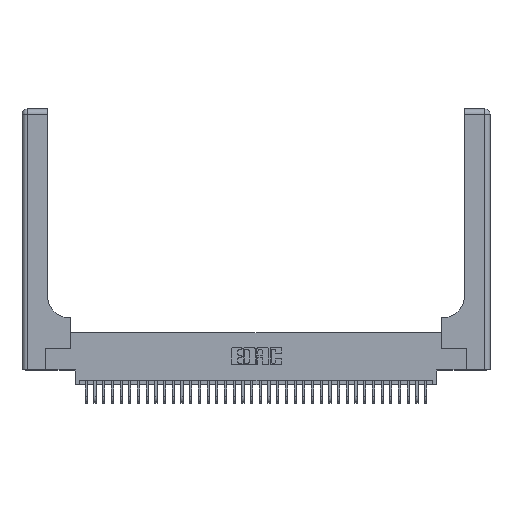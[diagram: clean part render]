
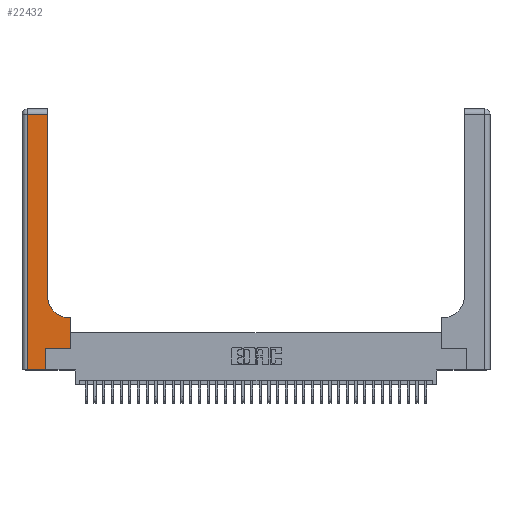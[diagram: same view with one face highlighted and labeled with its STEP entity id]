
A CAD part, top view. The second image highlights one B-rep face of the part: STEP entity #22432.
In plain terms, the highlighted planar face has unit normal (0, 0, 1).
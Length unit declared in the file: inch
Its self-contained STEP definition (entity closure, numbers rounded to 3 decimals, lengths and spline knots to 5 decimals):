
#737 = LINE ( 'NONE', #9791, #32551 ) ;
#1546 = VERTEX_POINT ( 'NONE', #38609 ) ;
#1738 = CARTESIAN_POINT ( 'NONE',  ( 0.5585, 0.25, 0.37 ) ) ;
#2170 = VERTEX_POINT ( 'NONE', #7391 ) ;
#2420 = ORIENTED_EDGE ( 'NONE', *, *, #10129, .T. ) ;
#2819 = CARTESIAN_POINT ( 'NONE',  ( 0., 3., 0.37 ) ) ;
#3541 = ORIENTED_EDGE ( 'NONE', *, *, #13930, .T. ) ;
#3680 = DIRECTION ( 'NONE',  ( -1., 0., 0. ) ) ;
#3943 = VECTOR ( 'NONE', #24016, 39.37008 ) ;
#4893 = LINE ( 'NONE', #12239, #3943 ) ;
#5303 = VECTOR ( 'NONE', #13798, 39.37008 ) ;
#5900 = DIRECTION ( 'NONE',  ( -1., 0., 0. ) ) ;
#5926 = EDGE_LOOP ( 'NONE', ( #15578, #2420, #13577, #8033, #20537, #35206, #3541, #31419, #14170 ) ) ;
#6678 = VECTOR ( 'NONE', #29207, 39.37008 ) ;
#7329 = AXIS2_PLACEMENT_3D ( 'NONE', #15722, #36368, #18679 ) ;
#7391 = CARTESIAN_POINT ( 'NONE',  ( 0.06, 0., 0.37 ) ) ;
#7452 = VERTEX_POINT ( 'NONE', #28634 ) ;
#7682 = CARTESIAN_POINT ( 'NONE',  ( 0.2915, 3., 0.37 ) ) ;
#8033 = ORIENTED_EDGE ( 'NONE', *, *, #23792, .T. ) ;
#9218 = CARTESIAN_POINT ( 'NONE',  ( 0.269, 0.25, 0.37 ) ) ;
#9411 = LINE ( 'NONE', #7682, #25226 ) ;
#9791 = CARTESIAN_POINT ( 'NONE',  ( 0., 2.94, 0.37 ) ) ;
#10129 = EDGE_CURVE ( 'NONE', #33311, #28318, #737, .T. ) ;
#11507 = CIRCLE ( 'NONE', #7329, 0.25 ) ;
#12239 = CARTESIAN_POINT ( 'NONE',  ( 0.269, 0., 0.37 ) ) ;
#13577 = ORIENTED_EDGE ( 'NONE', *, *, #18171, .T. ) ;
#13798 = DIRECTION ( 'NONE',  ( 0., 1., 0. ) ) ;
#13930 = EDGE_CURVE ( 'NONE', #38083, #7452, #28159, .T. ) ;
#14170 = ORIENTED_EDGE ( 'NONE', *, *, #38014, .T. ) ;
#14702 = LINE ( 'NONE', #26218, #6678 ) ;
#15578 = ORIENTED_EDGE ( 'NONE', *, *, #23328, .T. ) ;
#15722 = CARTESIAN_POINT ( 'NONE',  ( 0.5415, 0.85, 0.37 ) ) ;
#16207 = CARTESIAN_POINT ( 'NONE',  ( 0.06, 3., 0.37 ) ) ;
#17421 = CARTESIAN_POINT ( 'NONE',  ( 0.06, 2.94, 0.37 ) ) ;
#17654 = CARTESIAN_POINT ( 'NONE',  ( 0.269, 0., 0.37 ) ) ;
#18171 = EDGE_CURVE ( 'NONE', #28318, #2170, #29360, .T. ) ;
#18679 = DIRECTION ( 'NONE',  ( 1., 0., 0. ) ) ;
#18783 = CARTESIAN_POINT ( 'NONE',  ( 0.2915, 2.94, 0.37 ) ) ;
#18912 = FACE_OUTER_BOUND ( 'NONE', #5926, .T. ) ;
#19329 = CARTESIAN_POINT ( 'NONE',  ( 0.2915, 0.85, 0.37 ) ) ;
#20537 = ORIENTED_EDGE ( 'NONE', *, *, #20706, .T. ) ;
#20706 = EDGE_CURVE ( 'NONE', #37801, #31878, #4893, .T. ) ;
#20800 = PLANE ( 'NONE',  #38296 ) ;
#22432 = ADVANCED_FACE ( 'NONE', ( #18912 ), #20800, .F. ) ;
#22898 = DIRECTION ( 'NONE',  ( 1., 0., 0. ) ) ;
#23328 = EDGE_CURVE ( 'NONE', #32780, #33311, #9411, .T. ) ;
#23777 = DIRECTION ( 'NONE',  ( 0., 0., -1. ) ) ;
#23792 = EDGE_CURVE ( 'NONE', #2170, #37801, #32641, .T. ) ;
#24016 = DIRECTION ( 'NONE',  ( 0., 1., 0. ) ) ;
#24794 = VECTOR ( 'NONE', #22898, 39.37008 ) ;
#25226 = VECTOR ( 'NONE', #28510, 39.37008 ) ;
#26218 = CARTESIAN_POINT ( 'NONE',  ( 0.269, 0.25, 0.37 ) ) ;
#26902 = EDGE_CURVE ( 'NONE', #7452, #1546, #29617, .T. ) ;
#28159 = LINE ( 'NONE', #1738, #5303 ) ;
#28307 = EDGE_CURVE ( 'NONE', #31878, #38083, #14702, .T. ) ;
#28318 = VERTEX_POINT ( 'NONE', #17421 ) ;
#28510 = DIRECTION ( 'NONE',  ( 0., 1., 0. ) ) ;
#28634 = CARTESIAN_POINT ( 'NONE',  ( 0.5585, 0.6, 0.37 ) ) ;
#28653 = DIRECTION ( 'NONE',  ( -1., 0., 0. ) ) ;
#29207 = DIRECTION ( 'NONE',  ( 1., 0., 0. ) ) ;
#29360 = LINE ( 'NONE', #16207, #35342 ) ;
#29617 = LINE ( 'NONE', #34838, #36532 ) ;
#31419 = ORIENTED_EDGE ( 'NONE', *, *, #26902, .T. ) ;
#31878 = VERTEX_POINT ( 'NONE', #9218 ) ;
#32551 = VECTOR ( 'NONE', #3680, 39.37008 ) ;
#32641 = LINE ( 'NONE', #34659, #24794 ) ;
#32780 = VERTEX_POINT ( 'NONE', #19329 ) ;
#33311 = VERTEX_POINT ( 'NONE', #18783 ) ;
#33915 = DIRECTION ( 'NONE',  ( 0., -1., 0. ) ) ;
#34659 = CARTESIAN_POINT ( 'NONE',  ( 0., 0., 0.37 ) ) ;
#34838 = CARTESIAN_POINT ( 'NONE',  ( 0.2915, 0.6, 0.37 ) ) ;
#35206 = ORIENTED_EDGE ( 'NONE', *, *, #28307, .T. ) ;
#35342 = VECTOR ( 'NONE', #33915, 39.37008 ) ;
#36368 = DIRECTION ( 'NONE',  ( 0., 0., -1. ) ) ;
#36532 = VECTOR ( 'NONE', #28653, 39.37008 ) ;
#36620 = CARTESIAN_POINT ( 'NONE',  ( 0.5585, 0.25, 0.37 ) ) ;
#37801 = VERTEX_POINT ( 'NONE', #17654 ) ;
#38014 = EDGE_CURVE ( 'NONE', #1546, #32780, #11507, .T. ) ;
#38083 = VERTEX_POINT ( 'NONE', #36620 ) ;
#38296 = AXIS2_PLACEMENT_3D ( 'NONE', #2819, #23777, #5900 ) ;
#38609 = CARTESIAN_POINT ( 'NONE',  ( 0.5415, 0.6, 0.37 ) ) ;
